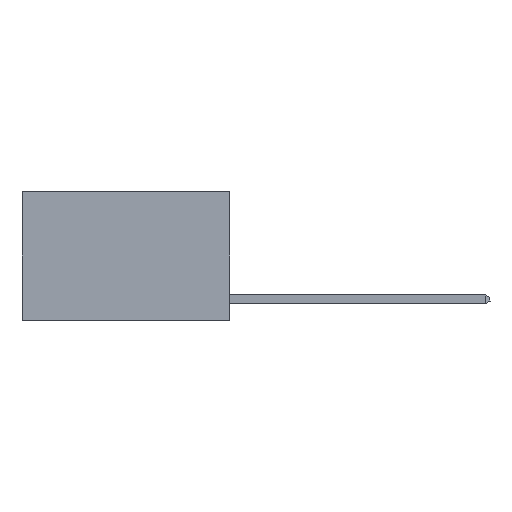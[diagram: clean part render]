
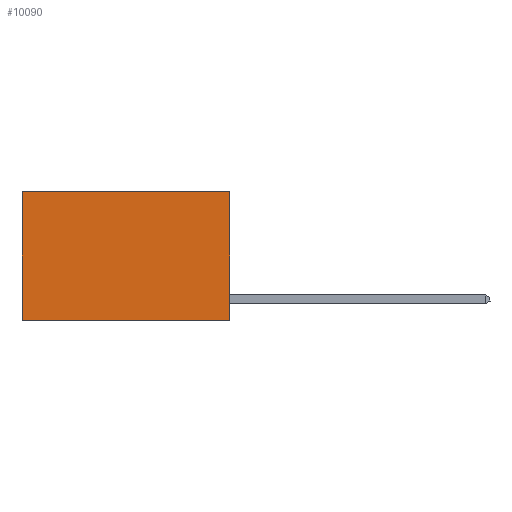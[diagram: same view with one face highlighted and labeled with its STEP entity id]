
A CAD part, left-side view. The second image highlights one B-rep face of the part: STEP entity #10090.
In plain terms, the highlighted planar face has unit normal (-1, 0, 0).
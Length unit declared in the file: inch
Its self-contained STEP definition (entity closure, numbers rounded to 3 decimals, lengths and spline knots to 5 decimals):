
#1897 = EDGE_CURVE ( 'NONE', #14106, #11919, #13514, .T. ) ;
#2023 = VERTEX_POINT ( 'NONE', #10321 ) ;
#3205 = EDGE_CURVE ( 'NONE', #6445, #14106, #8204, .T. ) ;
#4934 = PLANE ( 'NONE',  #13654 ) ;
#5452 = ORIENTED_EDGE ( 'NONE', *, *, #1897, .F. ) ;
#5532 = ORIENTED_EDGE ( 'NONE', *, *, #7411, .T. ) ;
#6197 = CARTESIAN_POINT ( 'NONE',  ( 0.2625, 0., 0. ) ) ;
#6265 = CARTESIAN_POINT ( 'NONE',  ( 0.2625, 0.6, -0.37 ) ) ;
#6378 = FACE_OUTER_BOUND ( 'NONE', #12922, .T. ) ;
#6445 = VERTEX_POINT ( 'NONE', #11620 ) ;
#7112 = VECTOR ( 'NONE', #9757, 39.37008 ) ;
#7411 = EDGE_CURVE ( 'NONE', #6445, #2023, #7443, .T. ) ;
#7439 = DIRECTION ( 'NONE',  ( 1., 0., 0. ) ) ;
#7443 = LINE ( 'NONE', #15961, #13453 ) ;
#8204 = LINE ( 'NONE', #15919, #14588 ) ;
#8429 = EDGE_CURVE ( 'NONE', #2023, #11919, #12525, .T. ) ;
#8459 = CARTESIAN_POINT ( 'NONE',  ( 0.2625, 0., -0.37 ) ) ;
#8815 = DIRECTION ( 'NONE',  ( 0., 0., -1. ) ) ;
#8998 = DIRECTION ( 'NONE',  ( 0., 0., -1. ) ) ;
#9757 = DIRECTION ( 'NONE',  ( 0., 1., 0. ) ) ;
#10090 = ADVANCED_FACE ( 'NONE', ( #6378 ), #4934, .F. ) ;
#10122 = DIRECTION ( 'NONE',  ( 0., 1., 0. ) ) ;
#10321 = CARTESIAN_POINT ( 'NONE',  ( 0.2625, 0.6, 0. ) ) ;
#10391 = ORIENTED_EDGE ( 'NONE', *, *, #3205, .F. ) ;
#11386 = CARTESIAN_POINT ( 'NONE',  ( 0.2625, 0.6, 0. ) ) ;
#11620 = CARTESIAN_POINT ( 'NONE',  ( 0.2625, 0., 0. ) ) ;
#11919 = VERTEX_POINT ( 'NONE', #6265 ) ;
#12113 = ORIENTED_EDGE ( 'NONE', *, *, #8429, .T. ) ;
#12525 = LINE ( 'NONE', #11386, #13056 ) ;
#12922 = EDGE_LOOP ( 'NONE', ( #12113, #5452, #10391, #5532 ) ) ;
#13027 = CARTESIAN_POINT ( 'NONE',  ( 0.2625, 0., -0.37 ) ) ;
#13056 = VECTOR ( 'NONE', #8998, 39.37008 ) ;
#13453 = VECTOR ( 'NONE', #10122, 39.37008 ) ;
#13514 = LINE ( 'NONE', #8459, #7112 ) ;
#13654 = AXIS2_PLACEMENT_3D ( 'NONE', #6197, #7439, #15791 ) ;
#14106 = VERTEX_POINT ( 'NONE', #13027 ) ;
#14588 = VECTOR ( 'NONE', #8815, 39.37008 ) ;
#15791 = DIRECTION ( 'NONE',  ( 0., 0., -1. ) ) ;
#15919 = CARTESIAN_POINT ( 'NONE',  ( 0.2625, 0., 0. ) ) ;
#15961 = CARTESIAN_POINT ( 'NONE',  ( 0.2625, 0., 0. ) ) ;
